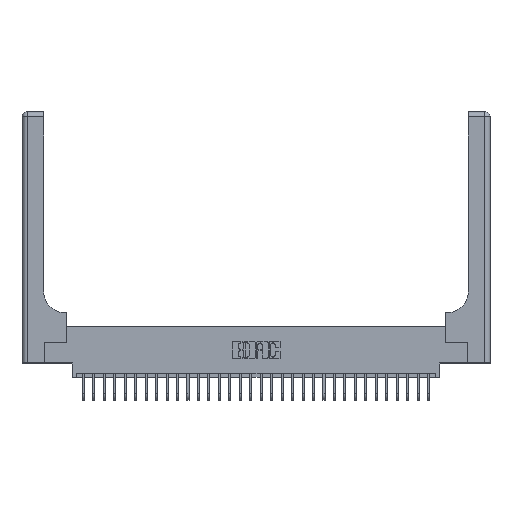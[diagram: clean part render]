
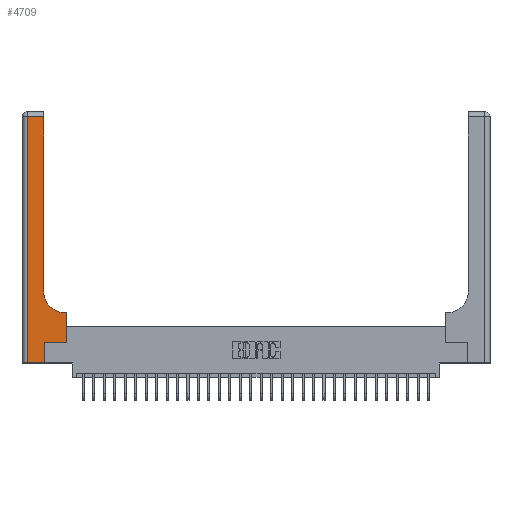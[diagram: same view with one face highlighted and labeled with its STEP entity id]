
A CAD part, top view. The second image highlights one B-rep face of the part: STEP entity #4709.
In plain terms, the highlighted planar face has unit normal (0, 0, 1).
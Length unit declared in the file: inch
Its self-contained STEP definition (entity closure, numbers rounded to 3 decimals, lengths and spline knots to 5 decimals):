
#1193 = CARTESIAN_POINT ( 'NONE',  ( 0.265, 0.25, 0.37 ) ) ;
#1840 = EDGE_CURVE ( 'NONE', #5987, #16360, #21478, .T. ) ;
#2940 = LINE ( 'NONE', #19616, #13071 ) ;
#3005 = VERTEX_POINT ( 'NONE', #26237 ) ;
#3278 = CARTESIAN_POINT ( 'NONE',  ( 0.06, 2.94, 0.37 ) ) ;
#3859 = CARTESIAN_POINT ( 'NONE',  ( 0.06, 0., 0.37 ) ) ;
#4478 = EDGE_CURVE ( 'NONE', #6814, #5987, #27931, .T. ) ;
#4709 = ADVANCED_FACE ( 'NONE', ( #19797 ), #24316, .F. ) ;
#4741 = EDGE_CURVE ( 'NONE', #16360, #17411, #21690, .T. ) ;
#4791 = VECTOR ( 'NONE', #19443, 39.37008 ) ;
#4792 = EDGE_LOOP ( 'NONE', ( #12645, #10404, #28827, #15958, #24054, #25808, #14226, #25776, #29361 ) ) ;
#5987 = VERTEX_POINT ( 'NONE', #17041 ) ;
#6414 = CARTESIAN_POINT ( 'NONE',  ( 0.528, 0.25, 0.37 ) ) ;
#6417 = VERTEX_POINT ( 'NONE', #24674 ) ;
#6814 = VERTEX_POINT ( 'NONE', #3859 ) ;
#7272 = AXIS2_PLACEMENT_3D ( 'NONE', #19335, #14796, #26499 ) ;
#7458 = DIRECTION ( 'NONE',  ( -1., 0., 0. ) ) ;
#7751 = DIRECTION ( 'NONE',  ( 0., 1., 0. ) ) ;
#8097 = DIRECTION ( 'NONE',  ( 1., 0., 0. ) ) ;
#8897 = CARTESIAN_POINT ( 'NONE',  ( 0., 0., 0.37 ) ) ;
#9268 = VECTOR ( 'NONE', #8097, 39.37008 ) ;
#9409 = VERTEX_POINT ( 'NONE', #14349 ) ;
#10404 = ORIENTED_EDGE ( 'NONE', *, *, #25750, .T. ) ;
#10771 = LINE ( 'NONE', #6414, #23955 ) ;
#10941 = EDGE_CURVE ( 'NONE', #3005, #22089, #28695, .T. ) ;
#11373 = EDGE_CURVE ( 'NONE', #20680, #6814, #24418, .T. ) ;
#12164 = DIRECTION ( 'NONE',  ( -1., 0., 0. ) ) ;
#12645 = ORIENTED_EDGE ( 'NONE', *, *, #29281, .T. ) ;
#13071 = VECTOR ( 'NONE', #7458, 39.37008 ) ;
#14226 = ORIENTED_EDGE ( 'NONE', *, *, #19027, .T. ) ;
#14349 = CARTESIAN_POINT ( 'NONE',  ( 0.26, 2.94, 0.37 ) ) ;
#14796 = DIRECTION ( 'NONE',  ( 0., 0., -1. ) ) ;
#15267 = DIRECTION ( 'NONE',  ( 0., 0., -1. ) ) ;
#15729 = CARTESIAN_POINT ( 'NONE',  ( 0.26, 0.85, 0.37 ) ) ;
#15918 = DIRECTION ( 'NONE',  ( 0., 1., 0. ) ) ;
#15958 = ORIENTED_EDGE ( 'NONE', *, *, #4478, .T. ) ;
#16360 = VERTEX_POINT ( 'NONE', #1193 ) ;
#16831 = DIRECTION ( 'NONE',  ( -1., 0., 0. ) ) ;
#17041 = CARTESIAN_POINT ( 'NONE',  ( 0.265, 0., 0.37 ) ) ;
#17410 = CARTESIAN_POINT ( 'NONE',  ( 0.265, 0., 0.37 ) ) ;
#17411 = VERTEX_POINT ( 'NONE', #29515 ) ;
#19027 = EDGE_CURVE ( 'NONE', #17411, #6417, #10771, .T. ) ;
#19147 = CARTESIAN_POINT ( 'NONE',  ( 0.06, 3., 0.37 ) ) ;
#19335 = CARTESIAN_POINT ( 'NONE',  ( 0.51, 0.85, 0.37 ) ) ;
#19443 = DIRECTION ( 'NONE',  ( 0., 1., 0. ) ) ;
#19613 = LINE ( 'NONE', #29135, #30101 ) ;
#19616 = CARTESIAN_POINT ( 'NONE',  ( 0.26, 0.6, 0.37 ) ) ;
#19735 = AXIS2_PLACEMENT_3D ( 'NONE', #27137, #15267, #12164 ) ;
#19797 = FACE_OUTER_BOUND ( 'NONE', #4792, .T. ) ;
#20680 = VERTEX_POINT ( 'NONE', #3278 ) ;
#21201 = EDGE_CURVE ( 'NONE', #6417, #3005, #2940, .T. ) ;
#21478 = LINE ( 'NONE', #17410, #4791 ) ;
#21690 = LINE ( 'NONE', #28875, #9268 ) ;
#21781 = VECTOR ( 'NONE', #29673, 39.37008 ) ;
#21944 = DIRECTION ( 'NONE',  ( 0., -1., 0. ) ) ;
#22089 = VERTEX_POINT ( 'NONE', #15729 ) ;
#23543 = VECTOR ( 'NONE', #16831, 39.37008 ) ;
#23955 = VECTOR ( 'NONE', #15918, 39.37008 ) ;
#24054 = ORIENTED_EDGE ( 'NONE', *, *, #1840, .T. ) ;
#24316 = PLANE ( 'NONE',  #19735 ) ;
#24418 = LINE ( 'NONE', #19147, #29720 ) ;
#24674 = CARTESIAN_POINT ( 'NONE',  ( 0.528, 0.6, 0.37 ) ) ;
#25750 = EDGE_CURVE ( 'NONE', #9409, #20680, #28396, .T. ) ;
#25776 = ORIENTED_EDGE ( 'NONE', *, *, #21201, .T. ) ;
#25808 = ORIENTED_EDGE ( 'NONE', *, *, #4741, .T. ) ;
#26237 = CARTESIAN_POINT ( 'NONE',  ( 0.51, 0.6, 0.37 ) ) ;
#26499 = DIRECTION ( 'NONE',  ( 1., 0., 0. ) ) ;
#27137 = CARTESIAN_POINT ( 'NONE',  ( 0., 3., 0.37 ) ) ;
#27931 = LINE ( 'NONE', #8897, #21781 ) ;
#28396 = LINE ( 'NONE', #30587, #23543 ) ;
#28695 = CIRCLE ( 'NONE', #7272, 0.25 ) ;
#28827 = ORIENTED_EDGE ( 'NONE', *, *, #11373, .T. ) ;
#28875 = CARTESIAN_POINT ( 'NONE',  ( 0.265, 0.25, 0.37 ) ) ;
#29135 = CARTESIAN_POINT ( 'NONE',  ( 0.26, 3., 0.37 ) ) ;
#29281 = EDGE_CURVE ( 'NONE', #22089, #9409, #19613, .T. ) ;
#29361 = ORIENTED_EDGE ( 'NONE', *, *, #10941, .T. ) ;
#29515 = CARTESIAN_POINT ( 'NONE',  ( 0.528, 0.25, 0.37 ) ) ;
#29673 = DIRECTION ( 'NONE',  ( 1., 0., 0. ) ) ;
#29720 = VECTOR ( 'NONE', #21944, 39.37008 ) ;
#30101 = VECTOR ( 'NONE', #7751, 39.37008 ) ;
#30587 = CARTESIAN_POINT ( 'NONE',  ( 0., 2.94, 0.37 ) ) ;
